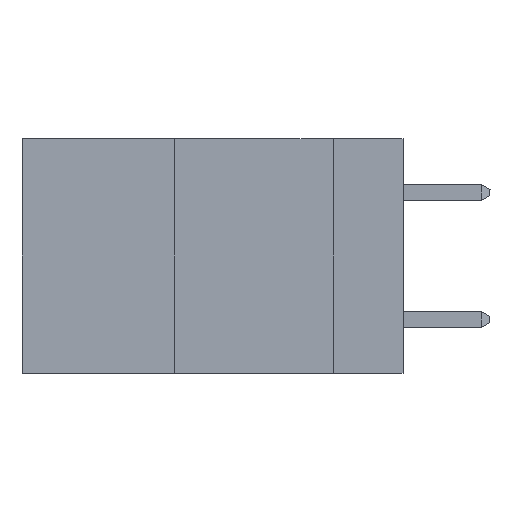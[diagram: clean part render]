
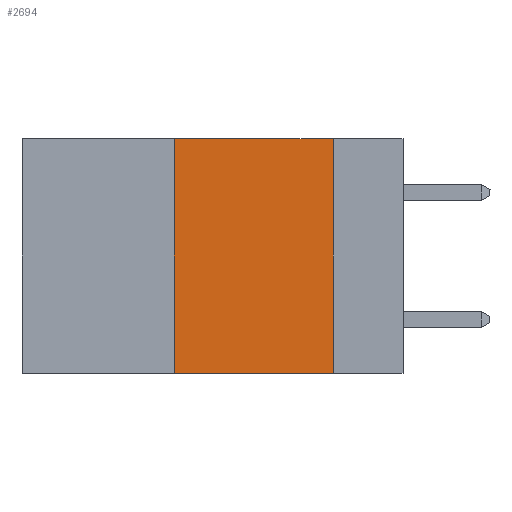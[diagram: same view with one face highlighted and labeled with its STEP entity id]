
A CAD part, left-side view. The second image highlights one B-rep face of the part: STEP entity #2694.
In plain terms, the highlighted planar face has unit normal (-1, 0, 0).
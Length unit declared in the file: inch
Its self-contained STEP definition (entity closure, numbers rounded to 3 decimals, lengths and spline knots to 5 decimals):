
#457 = CARTESIAN_POINT ( 'NONE',  ( 0., 0.36, 0. ) ) ;
#1295 = VECTOR ( 'NONE', #9979, 39.37008 ) ;
#1335 = PLANE ( 'NONE',  #12622 ) ;
#1385 = EDGE_CURVE ( 'NONE', #3036, #2125, #5047, .T. ) ;
#2125 = VERTEX_POINT ( 'NONE', #3498 ) ;
#2482 = CARTESIAN_POINT ( 'NONE',  ( 0., 0.6, 0. ) ) ;
#2694 = ADVANCED_FACE ( 'NONE', ( #10253 ), #1335, .F. ) ;
#3036 = VERTEX_POINT ( 'NONE', #6547 ) ;
#3187 = CARTESIAN_POINT ( 'NONE',  ( 0., 0.36, -0.37 ) ) ;
#3498 = CARTESIAN_POINT ( 'NONE',  ( 0., 0.11, 0. ) ) ;
#3642 = DIRECTION ( 'NONE',  ( 1., 0., 0. ) ) ;
#3891 = DIRECTION ( 'NONE',  ( 0., 0., -1. ) ) ;
#5047 = LINE ( 'NONE', #8844, #1295 ) ;
#5179 = ORIENTED_EDGE ( 'NONE', *, *, #6102, .F. ) ;
#6102 = EDGE_CURVE ( 'NONE', #2125, #14487, #11641, .T. ) ;
#6159 = VERTEX_POINT ( 'NONE', #3187 ) ;
#6547 = CARTESIAN_POINT ( 'NONE',  ( 0., 0.36, 0. ) ) ;
#6899 = VECTOR ( 'NONE', #10555, 39.37008 ) ;
#7274 = CARTESIAN_POINT ( 'NONE',  ( 0., 0.6, -0.37 ) ) ;
#7825 = CARTESIAN_POINT ( 'NONE',  ( 0., 0.11, -0.37 ) ) ;
#7953 = EDGE_CURVE ( 'NONE', #6159, #14487, #13183, .T. ) ;
#8844 = CARTESIAN_POINT ( 'NONE',  ( 0., 0.6, 0. ) ) ;
#9309 = DIRECTION ( 'NONE',  ( 0., 0., -1. ) ) ;
#9316 = ORIENTED_EDGE ( 'NONE', *, *, #1385, .F. ) ;
#9930 = ORIENTED_EDGE ( 'NONE', *, *, #12526, .F. ) ;
#9979 = DIRECTION ( 'NONE',  ( 0., -1., 0. ) ) ;
#10223 = VECTOR ( 'NONE', #12035, 39.37008 ) ;
#10253 = FACE_OUTER_BOUND ( 'NONE', #12674, .T. ) ;
#10555 = DIRECTION ( 'NONE',  ( 0., -1., 0. ) ) ;
#11304 = LINE ( 'NONE', #457, #10223 ) ;
#11638 = ORIENTED_EDGE ( 'NONE', *, *, #7953, .T. ) ;
#11641 = LINE ( 'NONE', #14875, #12541 ) ;
#12035 = DIRECTION ( 'NONE',  ( 0., 0., 1. ) ) ;
#12526 = EDGE_CURVE ( 'NONE', #6159, #3036, #11304, .T. ) ;
#12541 = VECTOR ( 'NONE', #9309, 39.37008 ) ;
#12622 = AXIS2_PLACEMENT_3D ( 'NONE', #2482, #3642, #3891 ) ;
#12674 = EDGE_LOOP ( 'NONE', ( #5179, #9316, #9930, #11638 ) ) ;
#13183 = LINE ( 'NONE', #7274, #6899 ) ;
#14487 = VERTEX_POINT ( 'NONE', #7825 ) ;
#14875 = CARTESIAN_POINT ( 'NONE',  ( 0., 0.11, 0. ) ) ;
